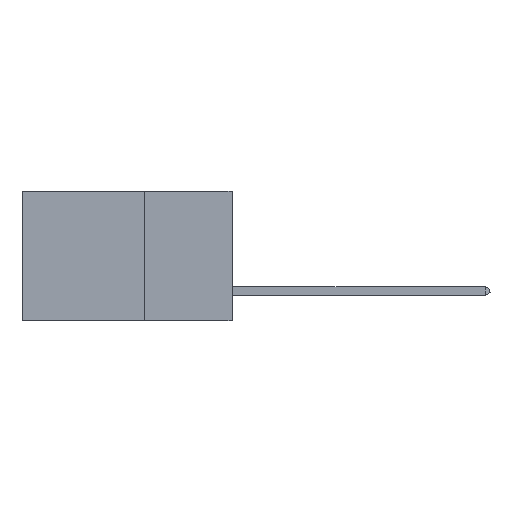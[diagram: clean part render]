
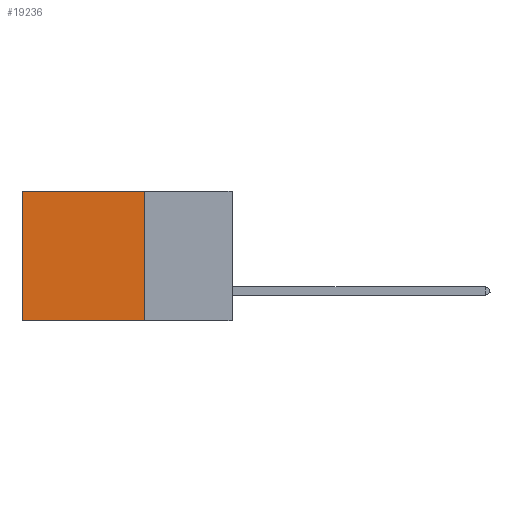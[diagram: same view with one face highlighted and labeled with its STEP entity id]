
A CAD part, left-side view. The second image highlights one B-rep face of the part: STEP entity #19236.
In plain terms, the highlighted planar face has unit normal (-1, 0, 0).
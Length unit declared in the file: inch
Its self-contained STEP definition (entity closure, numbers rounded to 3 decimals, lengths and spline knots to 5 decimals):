
#2 = EDGE_CURVE ( 'NONE', #30130, #34986, #25553, .T. ) ;
#238 = EDGE_LOOP ( 'NONE', ( #18094, #37770, #40859, #18429 ) ) ;
#3923 = EDGE_CURVE ( 'NONE', #19190, #17950, #42791, .T. ) ;
#5233 = EDGE_CURVE ( 'NONE', #30130, #19190, #25209, .T. ) ;
#5691 = VECTOR ( 'NONE', #28172, 39.37008 ) ;
#8629 = CARTESIAN_POINT ( 'NONE',  ( 0.2875, 0.6, 0. ) ) ;
#11630 = CARTESIAN_POINT ( 'NONE',  ( 0.2875, 0.6, 0. ) ) ;
#12221 = CARTESIAN_POINT ( 'NONE',  ( 0.2875, 0.25, 0. ) ) ;
#15716 = CARTESIAN_POINT ( 'NONE',  ( 0.2875, 0.25, 0. ) ) ;
#16465 = CARTESIAN_POINT ( 'NONE',  ( 0.2875, 0.25, -0.37 ) ) ;
#17046 = CARTESIAN_POINT ( 'NONE',  ( 0.2875, 0.25, 0. ) ) ;
#17950 = VERTEX_POINT ( 'NONE', #35505 ) ;
#18094 = ORIENTED_EDGE ( 'NONE', *, *, #41356, .T. ) ;
#18429 = ORIENTED_EDGE ( 'NONE', *, *, #2, .T. ) ;
#18692 = CARTESIAN_POINT ( 'NONE',  ( 0.2875, 0.25, -0.37 ) ) ;
#18866 = VECTOR ( 'NONE', #23858, 39.37008 ) ;
#19190 = VERTEX_POINT ( 'NONE', #18692 ) ;
#19236 = ADVANCED_FACE ( 'NONE', ( #25088 ), #45531, .F. ) ;
#22005 = VECTOR ( 'NONE', #23737, 39.37008 ) ;
#22948 = DIRECTION ( 'NONE',  ( 1., 0., 0. ) ) ;
#23737 = DIRECTION ( 'NONE',  ( 0., 1., 0. ) ) ;
#23858 = DIRECTION ( 'NONE',  ( 0., 0., -1. ) ) ;
#25088 = FACE_OUTER_BOUND ( 'NONE', #238, .T. ) ;
#25209 = LINE ( 'NONE', #35796, #31066 ) ;
#25553 = LINE ( 'NONE', #12221, #22005 ) ;
#28172 = DIRECTION ( 'NONE',  ( 0., 1., 0. ) ) ;
#28871 = LINE ( 'NONE', #8629, #18866 ) ;
#30130 = VERTEX_POINT ( 'NONE', #17046 ) ;
#30532 = DIRECTION ( 'NONE',  ( 0., 0., -1. ) ) ;
#31066 = VECTOR ( 'NONE', #32962, 39.37008 ) ;
#32511 = AXIS2_PLACEMENT_3D ( 'NONE', #15716, #22948, #30532 ) ;
#32962 = DIRECTION ( 'NONE',  ( 0., 0., -1. ) ) ;
#34986 = VERTEX_POINT ( 'NONE', #11630 ) ;
#35505 = CARTESIAN_POINT ( 'NONE',  ( 0.2875, 0.6, -0.37 ) ) ;
#35796 = CARTESIAN_POINT ( 'NONE',  ( 0.2875, 0.25, 0. ) ) ;
#37770 = ORIENTED_EDGE ( 'NONE', *, *, #3923, .F. ) ;
#40859 = ORIENTED_EDGE ( 'NONE', *, *, #5233, .F. ) ;
#41356 = EDGE_CURVE ( 'NONE', #34986, #17950, #28871, .T. ) ;
#42791 = LINE ( 'NONE', #16465, #5691 ) ;
#45531 = PLANE ( 'NONE',  #32511 ) ;
